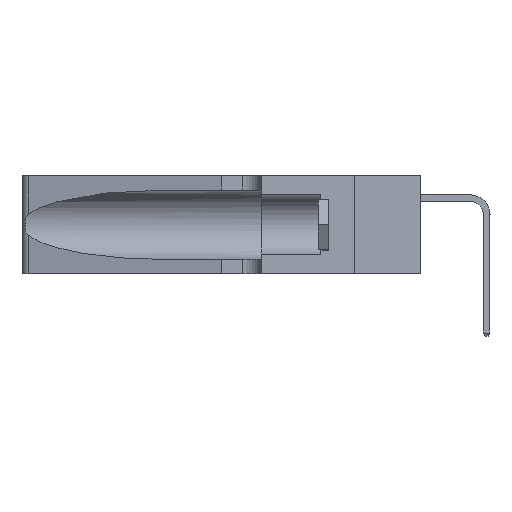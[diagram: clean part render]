
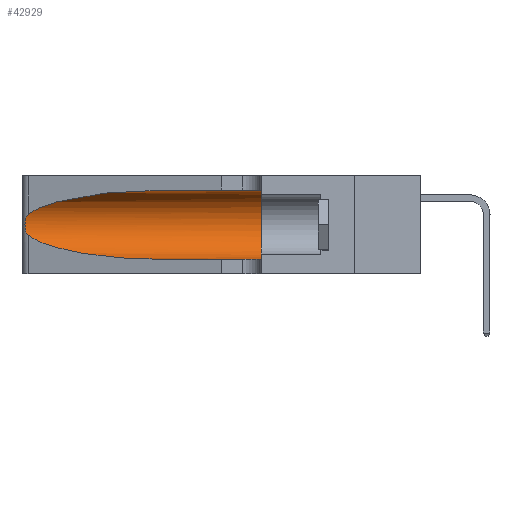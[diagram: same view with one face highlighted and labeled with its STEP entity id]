
A CAD part, left-side view. The second image highlights one B-rep face of the part: STEP entity #42929.
In plain terms, the highlighted cylindrical face has radius 3.308 mm (diameter 6.617 mm), a partial arc.
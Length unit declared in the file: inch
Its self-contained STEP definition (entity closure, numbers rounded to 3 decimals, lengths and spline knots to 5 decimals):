
#1373 = EDGE_CURVE ( 'NONE', #9646, #23940, #32855, .T. ) ;
#2655 = EDGE_CURVE ( 'NONE', #14113, #9646, #26513, .T. ) ;
#3293 = EDGE_CURVE ( 'NONE', #23940, #10257, #12962, .T. ) ;
#4508 = ORIENTED_EDGE ( 'NONE', *, *, #5232, .F. ) ;
#5106 = CARTESIAN_POINT ( 'NONE',  ( 0.25787, 1.23484, 0.2124 ) ) ;
#5232 = EDGE_CURVE ( 'NONE', #42601, #10257, #12241, .T. ) ;
#5768 = CARTESIAN_POINT ( 'NONE',  ( 0.1305, 0.35, 0.05475 ) ) ;
#7380 = CARTESIAN_POINT ( 'NONE',  ( 0.18966, 0.96281, 0.05475 ) ) ;
#7617 = CARTESIAN_POINT ( 'NONE',  ( 0.1305, 1.61858, 0.31525 ) ) ;
#7708 = DIRECTION ( 'NONE',  ( 0., -1., 0. ) ) ;
#8101 = CARTESIAN_POINT ( 'NONE',  ( 0.2373, 1.15595, 0.28018 ) ) ;
#8349 = CARTESIAN_POINT ( 'NONE',  ( 0.1305, 0.72297, 0.05475 ) ) ;
#8493 = CARTESIAN_POINT ( 'NONE',  ( 0.26018, 1.23835, 0.19895 ) ) ;
#8495 = EDGE_CURVE ( 'NONE', #24495, #42601, #17894, .T. ) ;
#9646 = VERTEX_POINT ( 'NONE', #10215 ) ;
#10215 = CARTESIAN_POINT ( 'NONE',  ( 0.25487, 1.22718, 0.14631 ) ) ;
#10257 = VERTEX_POINT ( 'NONE', #5768 ) ;
#10826 = CARTESIAN_POINT ( 'NONE',  ( 0.2373, 1.15595, 0.08982 ) ) ;
#11573 = ORIENTED_EDGE ( 'NONE', *, *, #16933, .T. ) ;
#11795 = CARTESIAN_POINT ( 'NONE',  ( 0.25555, 1.22994, 0.2215 ) ) ;
#11948 = CARTESIAN_POINT ( 'NONE',  ( 0.26075, 1.23896, 0.178 ) ) ;
#12241 = CIRCLE ( 'NONE', #35545, 0.13025 ) ;
#12962 = LINE ( 'NONE', #42756, #39285 ) ;
#14113 = VERTEX_POINT ( 'NONE', #23215 ) ;
#14368 = ORIENTED_EDGE ( 'NONE', *, *, #3293, .T. ) ;
#14454 = DIRECTION ( 'NONE',  ( 0., 0., -1. ) ) ;
#15401 = CARTESIAN_POINT ( 'NONE',  ( 0.25856, 1.23593, 0.16098 ) ) ;
#16933 = EDGE_CURVE ( 'NONE', #24495, #14113, #18437, .T. ) ;
#17441 = CARTESIAN_POINT ( 'NONE',  ( 0.1305, 0.72297, 0.05475 ) ) ;
#17568 = CARTESIAN_POINT ( 'NONE',  ( 0.1305, 0.35, 0.185 ) ) ;
#17894 = LINE ( 'NONE', #7617, #34003 ) ;
#18437 =( BOUNDED_CURVE ( )  B_SPLINE_CURVE ( 3, ( #25216, #28688, #8101, #32145 ),
 .UNSPECIFIED., .F., .F. ) 
 B_SPLINE_CURVE_WITH_KNOTS ( ( 4, 4 ),
 ( 1.5708, 2.84003 ),
 .UNSPECIFIED. ) 
 CURVE ( )  GEOMETRIC_REPRESENTATION_ITEM ( )  RATIONAL_B_SPLINE_CURVE ( ( 1., 0.87, 0.87, 1. ) ) 
 REPRESENTATION_ITEM ( '' )  );
#18689 = CARTESIAN_POINT ( 'NONE',  ( 0.25487, 1.22718, 0.22369 ) ) ;
#18847 = CARTESIAN_POINT ( 'NONE',  ( 0.25639, 1.23186, 0.15144 ) ) ;
#21020 = ORIENTED_EDGE ( 'NONE', *, *, #2655, .T. ) ;
#21041 = DIRECTION ( 'NONE',  ( 0., 0., 1. ) ) ;
#21506 = EDGE_LOOP ( 'NONE', ( #11573, #21020, #27420, #14368, #4508, #23064 ) ) ;
#22304 = CARTESIAN_POINT ( 'NONE',  ( 0.25487, 1.22718, 0.14631 ) ) ;
#22712 = FACE_OUTER_BOUND ( 'NONE', #21506, .T. ) ;
#23064 = ORIENTED_EDGE ( 'NONE', *, *, #8495, .F. ) ;
#23215 = CARTESIAN_POINT ( 'NONE',  ( 0.25487, 1.22718, 0.22369 ) ) ;
#23940 = VERTEX_POINT ( 'NONE', #17441 ) ;
#24495 = VERTEX_POINT ( 'NONE', #33909 ) ;
#24715 = DIRECTION ( 'NONE',  ( 0., -1., 0. ) ) ;
#25216 = CARTESIAN_POINT ( 'NONE',  ( 0.1305, 0.72297, 0.31525 ) ) ;
#25596 = CARTESIAN_POINT ( 'NONE',  ( 0.25639, 1.23184, 0.21858 ) ) ;
#26513 = B_SPLINE_CURVE_WITH_KNOTS ( 'NONE', 3,
 ( #18689, #11795, #25596, #5106, #29068, #8493, #32531, #11948, #35968, #15401, #39413, #18847, #42810, #22304 ),
 .UNSPECIFIED., .F., .F.,
 ( 4, 2, 2, 2, 2, 2, 4 ),
 ( 0., 0.00027, 0.00053, 0.00107, 0.0016, 0.00187, 0.00214 ),
 .UNSPECIFIED. ) ;
#27420 = ORIENTED_EDGE ( 'NONE', *, *, #1373, .T. ) ;
#28688 = CARTESIAN_POINT ( 'NONE',  ( 0.18966, 0.96281, 0.31525 ) ) ;
#29068 = CARTESIAN_POINT ( 'NONE',  ( 0.25854, 1.2359, 0.20912 ) ) ;
#29164 = DIRECTION ( 'NONE',  ( 0., -1., 0. ) ) ;
#31734 = CARTESIAN_POINT ( 'NONE',  ( 0.1305, 1.61858, 0.185 ) ) ;
#32038 = AXIS2_PLACEMENT_3D ( 'NONE', #31734, #7708, #14454 ) ;
#32145 = CARTESIAN_POINT ( 'NONE',  ( 0.25487, 1.22718, 0.22369 ) ) ;
#32531 = CARTESIAN_POINT ( 'NONE',  ( 0.26075, 1.23896, 0.19203 ) ) ;
#32855 =( BOUNDED_CURVE ( )  B_SPLINE_CURVE ( 3, ( #40424, #10826, #7380, #8349 ),
 .UNSPECIFIED., .F., .F. ) 
 B_SPLINE_CURVE_WITH_KNOTS ( ( 4, 4 ),
 ( 3.44316, 4.71239 ),
 .UNSPECIFIED. ) 
 CURVE ( )  GEOMETRIC_REPRESENTATION_ITEM ( )  RATIONAL_B_SPLINE_CURVE ( ( 1., 0.87, 0.87, 1. ) ) 
 REPRESENTATION_ITEM ( '' )  );
#33909 = CARTESIAN_POINT ( 'NONE',  ( 0.1305, 0.72297, 0.31525 ) ) ;
#34003 = VECTOR ( 'NONE', #24715, 39.37008 ) ;
#35545 = AXIS2_PLACEMENT_3D ( 'NONE', #17568, #41551, #21041 ) ;
#35968 = CARTESIAN_POINT ( 'NONE',  ( 0.26017, 1.23833, 0.17102 ) ) ;
#37183 = CARTESIAN_POINT ( 'NONE',  ( 0.1305, 0.35, 0.31525 ) ) ;
#37757 = CYLINDRICAL_SURFACE ( 'NONE', #32038, 0.13025 ) ;
#39285 = VECTOR ( 'NONE', #29164, 39.37008 ) ;
#39413 = CARTESIAN_POINT ( 'NONE',  ( 0.25789, 1.23486, 0.15765 ) ) ;
#40424 = CARTESIAN_POINT ( 'NONE',  ( 0.25487, 1.22718, 0.14631 ) ) ;
#41551 = DIRECTION ( 'NONE',  ( 0., 1., 0. ) ) ;
#42601 = VERTEX_POINT ( 'NONE', #37183 ) ;
#42756 = CARTESIAN_POINT ( 'NONE',  ( 0.1305, 1.61858, 0.05475 ) ) ;
#42810 = CARTESIAN_POINT ( 'NONE',  ( 0.25555, 1.22993, 0.14849 ) ) ;
#42929 = ADVANCED_FACE ( 'NONE', ( #22712 ), #37757, .F. ) ;
